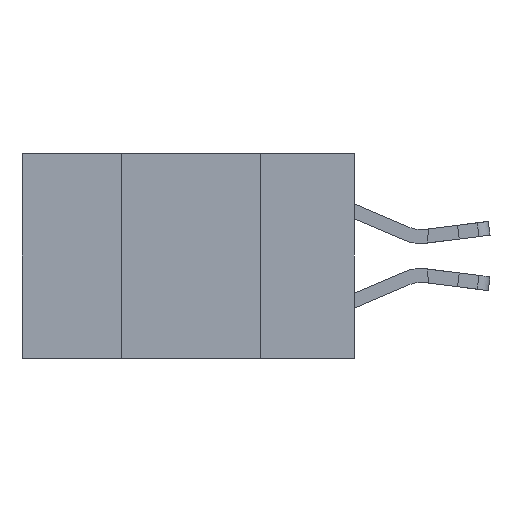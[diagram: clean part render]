
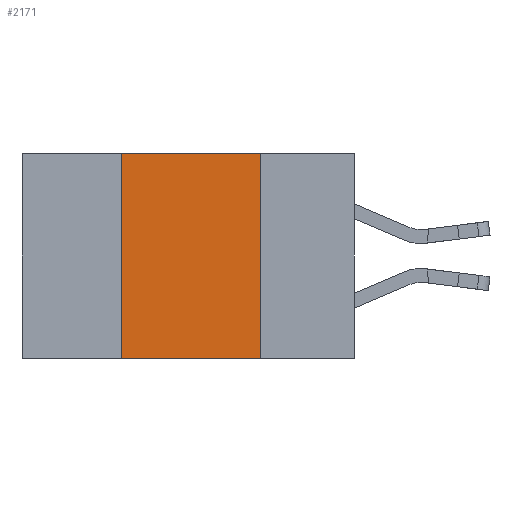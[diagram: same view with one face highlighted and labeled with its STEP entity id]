
A CAD part, left-side view. The second image highlights one B-rep face of the part: STEP entity #2171.
In plain terms, the highlighted planar face has unit normal (-1, 0, 0).
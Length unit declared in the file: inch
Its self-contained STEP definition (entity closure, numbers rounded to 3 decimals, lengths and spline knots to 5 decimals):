
#786 = FACE_OUTER_BOUND ( 'NONE', #10800, .T. ) ;
#1180 = VERTEX_POINT ( 'NONE', #9546 ) ;
#1605 = DIRECTION ( 'NONE',  ( 0., 0., 1. ) ) ;
#1824 = CARTESIAN_POINT ( 'NONE',  ( 0., 0.17, -0.37 ) ) ;
#1930 = DIRECTION ( 'NONE',  ( 0., 0., -1. ) ) ;
#2034 = PLANE ( 'NONE',  #8224 ) ;
#2040 = CARTESIAN_POINT ( 'NONE',  ( 0., 0.17, 0. ) ) ;
#2171 = ADVANCED_FACE ( 'NONE', ( #786 ), #2034, .F. ) ;
#2908 = ORIENTED_EDGE ( 'NONE', *, *, #12823, .F. ) ;
#4445 = VERTEX_POINT ( 'NONE', #9750 ) ;
#4841 = VECTOR ( 'NONE', #9390, 39.37008 ) ;
#4993 = LINE ( 'NONE', #2040, #10463 ) ;
#5497 = DIRECTION ( 'NONE',  ( 0., 0., -1. ) ) ;
#5696 = CARTESIAN_POINT ( 'NONE',  ( 0., 0.6, 0. ) ) ;
#6173 = VECTOR ( 'NONE', #11920, 39.37008 ) ;
#6922 = LINE ( 'NONE', #14012, #4841 ) ;
#6941 = VERTEX_POINT ( 'NONE', #1824 ) ;
#6993 = ORIENTED_EDGE ( 'NONE', *, *, #9584, .F. ) ;
#7258 = ORIENTED_EDGE ( 'NONE', *, *, #12418, .F. ) ;
#8036 = VERTEX_POINT ( 'NONE', #11986 ) ;
#8224 = AXIS2_PLACEMENT_3D ( 'NONE', #5696, #15047, #1930 ) ;
#9078 = LINE ( 'NONE', #14716, #14299 ) ;
#9390 = DIRECTION ( 'NONE',  ( 0., -1., 0. ) ) ;
#9546 = CARTESIAN_POINT ( 'NONE',  ( 0., 0.17, 0. ) ) ;
#9561 = CARTESIAN_POINT ( 'NONE',  ( 0., 0.6, -0.37 ) ) ;
#9584 = EDGE_CURVE ( 'NONE', #8036, #4445, #9078, .T. ) ;
#9639 = ORIENTED_EDGE ( 'NONE', *, *, #12218, .T. ) ;
#9732 = LINE ( 'NONE', #9561, #6173 ) ;
#9750 = CARTESIAN_POINT ( 'NONE',  ( 0., 0.42, 0. ) ) ;
#10463 = VECTOR ( 'NONE', #5497, 39.37008 ) ;
#10800 = EDGE_LOOP ( 'NONE', ( #2908, #7258, #6993, #9639 ) ) ;
#11920 = DIRECTION ( 'NONE',  ( 0., -1., 0. ) ) ;
#11986 = CARTESIAN_POINT ( 'NONE',  ( 0., 0.42, -0.37 ) ) ;
#12218 = EDGE_CURVE ( 'NONE', #8036, #6941, #9732, .T. ) ;
#12418 = EDGE_CURVE ( 'NONE', #4445, #1180, #6922, .T. ) ;
#12823 = EDGE_CURVE ( 'NONE', #1180, #6941, #4993, .T. ) ;
#14012 = CARTESIAN_POINT ( 'NONE',  ( 0., 0.6, 0. ) ) ;
#14299 = VECTOR ( 'NONE', #1605, 39.37008 ) ;
#14716 = CARTESIAN_POINT ( 'NONE',  ( 0., 0.42, 0. ) ) ;
#15047 = DIRECTION ( 'NONE',  ( 1., 0., 0. ) ) ;
